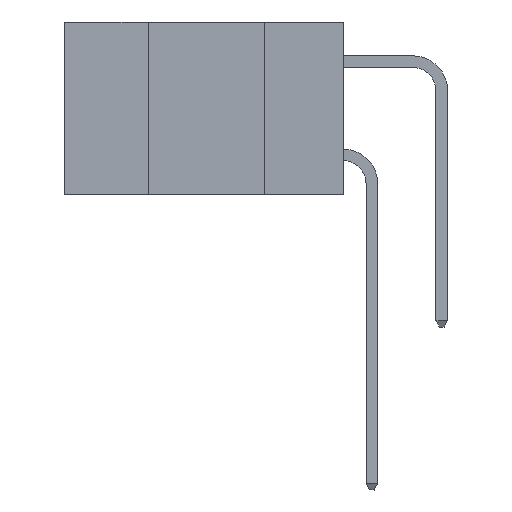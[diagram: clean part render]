
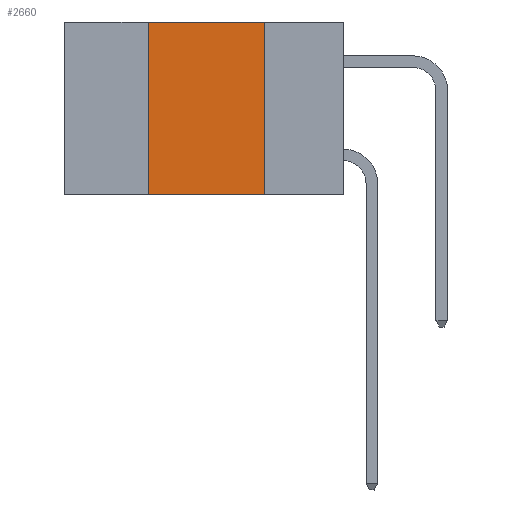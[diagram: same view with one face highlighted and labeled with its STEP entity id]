
A CAD part, left-side view. The second image highlights one B-rep face of the part: STEP entity #2660.
In plain terms, the highlighted planar face has unit normal (-1, 0, 0).
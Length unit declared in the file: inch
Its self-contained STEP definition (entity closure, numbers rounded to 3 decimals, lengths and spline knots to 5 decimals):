
#253 = CARTESIAN_POINT ( 'NONE',  ( 0., 0.42, -0.37 ) ) ;
#759 = DIRECTION ( 'NONE',  ( 0., 0., -1. ) ) ;
#793 = ORIENTED_EDGE ( 'NONE', *, *, #5463, .F. ) ;
#1078 = DIRECTION ( 'NONE',  ( 0., -1., 0. ) ) ;
#1103 = VERTEX_POINT ( 'NONE', #8194 ) ;
#1380 = ORIENTED_EDGE ( 'NONE', *, *, #4954, .F. ) ;
#1657 = CARTESIAN_POINT ( 'NONE',  ( 0., 0.6, 0. ) ) ;
#1778 = VECTOR ( 'NONE', #2115, 39.37008 ) ;
#2115 = DIRECTION ( 'NONE',  ( 0., -1., 0. ) ) ;
#2660 = ADVANCED_FACE ( 'NONE', ( #3718 ), #8926, .F. ) ;
#2996 = ORIENTED_EDGE ( 'NONE', *, *, #6549, .F. ) ;
#3120 = VERTEX_POINT ( 'NONE', #4811 ) ;
#3292 = VECTOR ( 'NONE', #1078, 39.37008 ) ;
#3424 = DIRECTION ( 'NONE',  ( 0., 0., 1. ) ) ;
#3718 = FACE_OUTER_BOUND ( 'NONE', #9025, .T. ) ;
#4766 = DIRECTION ( 'NONE',  ( 1., 0., 0. ) ) ;
#4811 = CARTESIAN_POINT ( 'NONE',  ( 0., 0.17, -0.37 ) ) ;
#4954 = EDGE_CURVE ( 'NONE', #8969, #7525, #5376, .T. ) ;
#5376 = LINE ( 'NONE', #253, #10711 ) ;
#5463 = EDGE_CURVE ( 'NONE', #1103, #3120, #9142, .T. ) ;
#6549 = EDGE_CURVE ( 'NONE', #7525, #1103, #7363, .T. ) ;
#7042 = CARTESIAN_POINT ( 'NONE',  ( 0., 0.17, -0.37 ) ) ;
#7363 = LINE ( 'NONE', #10476, #3292 ) ;
#7484 = CARTESIAN_POINT ( 'NONE',  ( 0., 0.6, -0.37 ) ) ;
#7525 = VERTEX_POINT ( 'NONE', #11976 ) ;
#7833 = EDGE_CURVE ( 'NONE', #8969, #3120, #12529, .T. ) ;
#7860 = VECTOR ( 'NONE', #759, 39.37008 ) ;
#8194 = CARTESIAN_POINT ( 'NONE',  ( 0., 0.17, 0. ) ) ;
#8926 = PLANE ( 'NONE',  #11703 ) ;
#8969 = VERTEX_POINT ( 'NONE', #10751 ) ;
#9025 = EDGE_LOOP ( 'NONE', ( #793, #2996, #1380, #13481 ) ) ;
#9142 = LINE ( 'NONE', #7042, #7860 ) ;
#10476 = CARTESIAN_POINT ( 'NONE',  ( 0., 0.6, 0. ) ) ;
#10711 = VECTOR ( 'NONE', #3424, 39.37008 ) ;
#10751 = CARTESIAN_POINT ( 'NONE',  ( 0., 0.42, -0.37 ) ) ;
#11703 = AXIS2_PLACEMENT_3D ( 'NONE', #1657, #4766, #13151 ) ;
#11976 = CARTESIAN_POINT ( 'NONE',  ( 0., 0.42, 0. ) ) ;
#12529 = LINE ( 'NONE', #7484, #1778 ) ;
#13151 = DIRECTION ( 'NONE',  ( 0., 0., -1. ) ) ;
#13481 = ORIENTED_EDGE ( 'NONE', *, *, #7833, .T. ) ;
